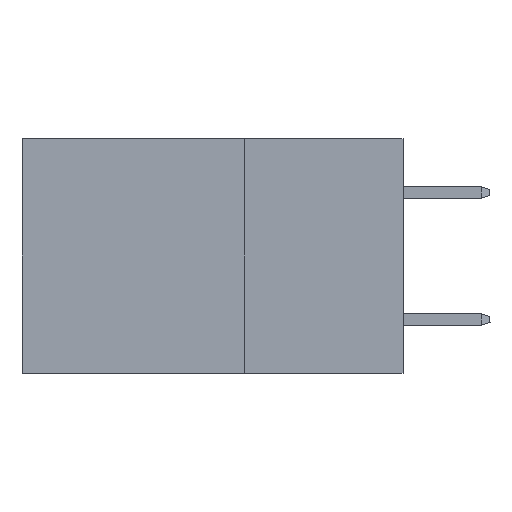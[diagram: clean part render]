
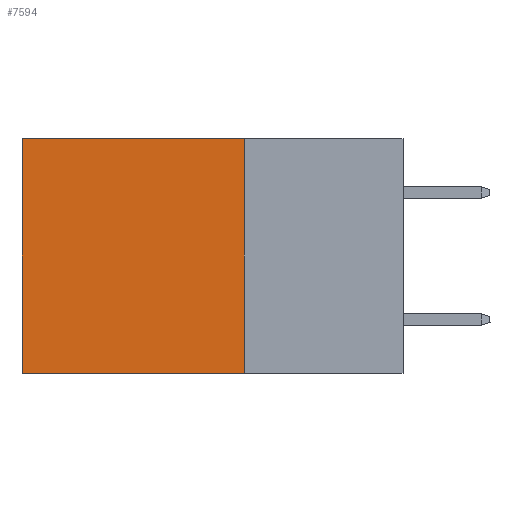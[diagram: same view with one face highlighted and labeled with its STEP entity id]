
A CAD part, left-side view. The second image highlights one B-rep face of the part: STEP entity #7594.
In plain terms, the highlighted planar face has unit normal (-1, 0, 0).
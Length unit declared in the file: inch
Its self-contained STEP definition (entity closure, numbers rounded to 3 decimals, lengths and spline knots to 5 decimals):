
#186 = CARTESIAN_POINT ( 'NONE',  ( 0.2875, 0.6, -0.37 ) ) ;
#364 = VECTOR ( 'NONE', #2417, 39.37008 ) ;
#1063 = ORIENTED_EDGE ( 'NONE', *, *, #10654, .T. ) ;
#1834 = LINE ( 'NONE', #9721, #4662 ) ;
#2396 = CARTESIAN_POINT ( 'NONE',  ( 0.2875, 0.25, -0.37 ) ) ;
#2417 = DIRECTION ( 'NONE',  ( 0., 1., 0. ) ) ;
#2486 = VERTEX_POINT ( 'NONE', #7592 ) ;
#3558 = VERTEX_POINT ( 'NONE', #2396 ) ;
#3730 = CARTESIAN_POINT ( 'NONE',  ( 0.2875, 0.6, 0. ) ) ;
#3920 = EDGE_CURVE ( 'NONE', #11725, #8991, #11886, .T. ) ;
#3978 = AXIS2_PLACEMENT_3D ( 'NONE', #11377, #12176, #9024 ) ;
#4094 = DIRECTION ( 'NONE',  ( 0., 0., -1. ) ) ;
#4312 = DIRECTION ( 'NONE',  ( 0., 0., -1. ) ) ;
#4662 = VECTOR ( 'NONE', #4312, 39.37008 ) ;
#4740 = PLANE ( 'NONE',  #3978 ) ;
#4913 = EDGE_LOOP ( 'NONE', ( #11169, #8783, #5519, #1063 ) ) ;
#5319 = CARTESIAN_POINT ( 'NONE',  ( 0.2875, 0.6, 0. ) ) ;
#5519 = ORIENTED_EDGE ( 'NONE', *, *, #5945, .F. ) ;
#5535 = LINE ( 'NONE', #7894, #12994 ) ;
#5945 = EDGE_CURVE ( 'NONE', #2486, #3558, #1834, .T. ) ;
#7592 = CARTESIAN_POINT ( 'NONE',  ( 0.2875, 0.25, 0. ) ) ;
#7594 = ADVANCED_FACE ( 'NONE', ( #7976 ), #4740, .F. ) ;
#7894 = CARTESIAN_POINT ( 'NONE',  ( 0.2875, 0.25, 0. ) ) ;
#7976 = FACE_OUTER_BOUND ( 'NONE', #4913, .T. ) ;
#8783 = ORIENTED_EDGE ( 'NONE', *, *, #10694, .F. ) ;
#8991 = VERTEX_POINT ( 'NONE', #186 ) ;
#9024 = DIRECTION ( 'NONE',  ( 0., 0., -1. ) ) ;
#9721 = CARTESIAN_POINT ( 'NONE',  ( 0.2875, 0.25, 0. ) ) ;
#10654 = EDGE_CURVE ( 'NONE', #2486, #11725, #5535, .T. ) ;
#10694 = EDGE_CURVE ( 'NONE', #3558, #8991, #11148, .T. ) ;
#11148 = LINE ( 'NONE', #12239, #364 ) ;
#11169 = ORIENTED_EDGE ( 'NONE', *, *, #3920, .T. ) ;
#11377 = CARTESIAN_POINT ( 'NONE',  ( 0.2875, 0.25, 0. ) ) ;
#11725 = VERTEX_POINT ( 'NONE', #3730 ) ;
#11779 = VECTOR ( 'NONE', #4094, 39.37008 ) ;
#11886 = LINE ( 'NONE', #5319, #11779 ) ;
#12170 = DIRECTION ( 'NONE',  ( 0., 1., 0. ) ) ;
#12176 = DIRECTION ( 'NONE',  ( 1., 0., 0. ) ) ;
#12239 = CARTESIAN_POINT ( 'NONE',  ( 0.2875, 0.25, -0.37 ) ) ;
#12994 = VECTOR ( 'NONE', #12170, 39.37008 ) ;
